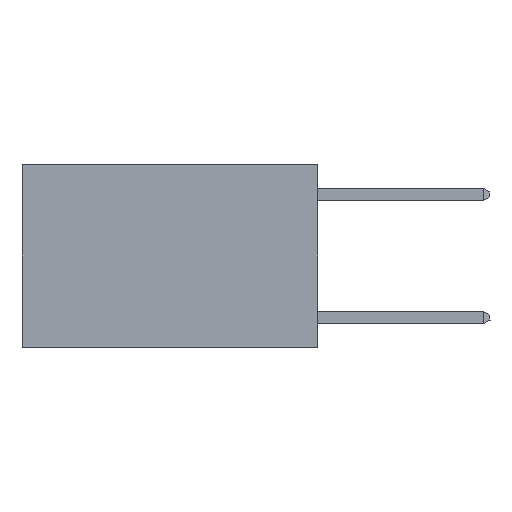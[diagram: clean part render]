
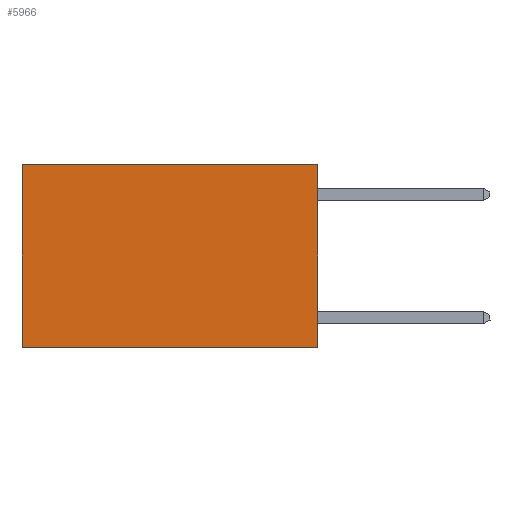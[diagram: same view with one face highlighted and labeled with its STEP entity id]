
A CAD part, left-side view. The second image highlights one B-rep face of the part: STEP entity #5966.
In plain terms, the highlighted planar face has unit normal (-1, 0, 0).
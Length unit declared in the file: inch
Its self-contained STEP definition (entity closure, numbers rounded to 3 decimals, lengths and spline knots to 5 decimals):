
#274 = EDGE_CURVE ( 'NONE', #1097, #23876, #875, .T. ) ;
#866 = CARTESIAN_POINT ( 'NONE',  ( 0.2625, 0.6, 0. ) ) ;
#875 = LINE ( 'NONE', #9001, #20576 ) ;
#880 = DIRECTION ( 'NONE',  ( 1., 0., 0. ) ) ;
#1097 = VERTEX_POINT ( 'NONE', #9049 ) ;
#1754 = VERTEX_POINT ( 'NONE', #12924 ) ;
#1781 = VECTOR ( 'NONE', #2923, 39.37008 ) ;
#2923 = DIRECTION ( 'NONE',  ( 0., 0., -1. ) ) ;
#3320 = VECTOR ( 'NONE', #18131, 39.37008 ) ;
#4467 = LINE ( 'NONE', #12184, #19503 ) ;
#5325 = AXIS2_PLACEMENT_3D ( 'NONE', #24152, #880, #14855 ) ;
#5966 = ADVANCED_FACE ( 'NONE', ( #9937 ), #22347, .F. ) ;
#7391 = ORIENTED_EDGE ( 'NONE', *, *, #17722, .T. ) ;
#8187 = VERTEX_POINT ( 'NONE', #21311 ) ;
#8353 = LINE ( 'NONE', #866, #1781 ) ;
#8357 = CARTESIAN_POINT ( 'NONE',  ( 0.2625, 0., 0. ) ) ;
#9001 = CARTESIAN_POINT ( 'NONE',  ( 0.2625, 0., -0.37 ) ) ;
#9049 = CARTESIAN_POINT ( 'NONE',  ( 0.2625, 0., -0.37 ) ) ;
#9937 = FACE_OUTER_BOUND ( 'NONE', #14688, .T. ) ;
#12184 = CARTESIAN_POINT ( 'NONE',  ( 0.2625, 0., 0. ) ) ;
#12924 = CARTESIAN_POINT ( 'NONE',  ( 0.2625, 0.6, 0. ) ) ;
#14688 = EDGE_LOOP ( 'NONE', ( #22778, #17391, #22652, #7391 ) ) ;
#14855 = DIRECTION ( 'NONE',  ( 0., 0., -1. ) ) ;
#15510 = EDGE_CURVE ( 'NONE', #8187, #1097, #18451, .T. ) ;
#16063 = DIRECTION ( 'NONE',  ( 0., 1., 0. ) ) ;
#17391 = ORIENTED_EDGE ( 'NONE', *, *, #274, .F. ) ;
#17722 = EDGE_CURVE ( 'NONE', #8187, #1754, #4467, .T. ) ;
#18131 = DIRECTION ( 'NONE',  ( 0., 0., -1. ) ) ;
#18451 = LINE ( 'NONE', #8357, #3320 ) ;
#19503 = VECTOR ( 'NONE', #16063, 39.37008 ) ;
#20576 = VECTOR ( 'NONE', #23459, 39.37008 ) ;
#20936 = EDGE_CURVE ( 'NONE', #1754, #23876, #8353, .T. ) ;
#21311 = CARTESIAN_POINT ( 'NONE',  ( 0.2625, 0., 0. ) ) ;
#22347 = PLANE ( 'NONE',  #5325 ) ;
#22652 = ORIENTED_EDGE ( 'NONE', *, *, #15510, .F. ) ;
#22778 = ORIENTED_EDGE ( 'NONE', *, *, #20936, .T. ) ;
#23459 = DIRECTION ( 'NONE',  ( 0., 1., 0. ) ) ;
#23538 = CARTESIAN_POINT ( 'NONE',  ( 0.2625, 0.6, -0.37 ) ) ;
#23876 = VERTEX_POINT ( 'NONE', #23538 ) ;
#24152 = CARTESIAN_POINT ( 'NONE',  ( 0.2625, 0., 0. ) ) ;
